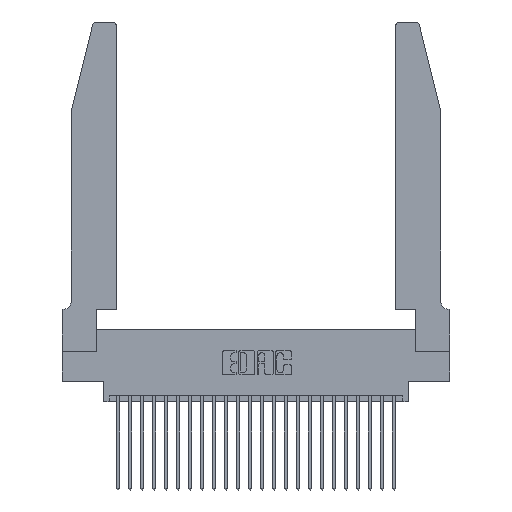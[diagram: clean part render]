
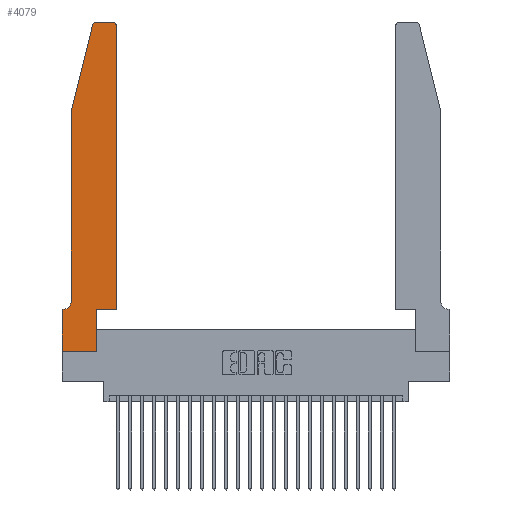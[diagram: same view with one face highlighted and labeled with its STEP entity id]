
A CAD part, top view. The second image highlights one B-rep face of the part: STEP entity #4079.
In plain terms, the highlighted planar face has unit normal (0, 0, 1).
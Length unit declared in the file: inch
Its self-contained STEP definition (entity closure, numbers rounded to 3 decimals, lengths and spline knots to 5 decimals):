
#277 = CIRCLE ( 'NONE', #853, 0.03 ) ;
#733 = CARTESIAN_POINT ( 'NONE',  ( 0.0755, 2., 0.37 ) ) ;
#740 = EDGE_CURVE ( 'NONE', #6446, #15986, #9805, .T. ) ;
#853 = AXIS2_PLACEMENT_3D ( 'NONE', #8101, #22144, #10156 ) ;
#1047 = LINE ( 'NONE', #12649, #11357 ) ;
#1340 = EDGE_CURVE ( 'NONE', #5785, #18816, #2372, .T. ) ;
#1494 = CARTESIAN_POINT ( 'NONE',  ( 0., 0., 0.37 ) ) ;
#1659 = LINE ( 'NONE', #18973, #11961 ) ;
#1955 = CARTESIAN_POINT ( 'NONE',  ( 0.4505, 2.72, 0.37 ) ) ;
#2372 = LINE ( 'NONE', #25134, #22603 ) ;
#2872 = CARTESIAN_POINT ( 'NONE',  ( 0.0755, 0.42, 0.37 ) ) ;
#3202 = CARTESIAN_POINT ( 'NONE',  ( 0., 0., 0.37 ) ) ;
#3206 = ORIENTED_EDGE ( 'NONE', *, *, #18783, .T. ) ;
#3615 = DIRECTION ( 'NONE',  ( 0., -1., 0. ) ) ;
#3975 = DIRECTION ( 'NONE',  ( 0., 0., -1. ) ) ;
#4079 = ADVANCED_FACE ( 'NONE', ( #21241 ), #5989, .T. ) ;
#4117 = EDGE_CURVE ( 'NONE', #4868, #4806, #277, .T. ) ;
#4322 = EDGE_CURVE ( 'NONE', #16030, #5785, #10305, .T. ) ;
#4368 = VECTOR ( 'NONE', #5799, 39.37008 ) ;
#4564 = CARTESIAN_POINT ( 'NONE',  ( 0.4205, 2.75, 0.37 ) ) ;
#4806 = VERTEX_POINT ( 'NONE', #12004 ) ;
#4868 = VERTEX_POINT ( 'NONE', #6229 ) ;
#5072 = AXIS2_PLACEMENT_3D ( 'NONE', #20044, #10072, #24035 ) ;
#5785 = VERTEX_POINT ( 'NONE', #21246 ) ;
#5799 = DIRECTION ( 'NONE',  ( 1., 0., 0. ) ) ;
#5846 = ORIENTED_EDGE ( 'NONE', *, *, #1340, .T. ) ;
#5989 = PLANE ( 'NONE',  #5072 ) ;
#6053 = CIRCLE ( 'NONE', #14151, 0.03 ) ;
#6054 = CARTESIAN_POINT ( 'NONE',  ( 0., 0.35, 0.37 ) ) ;
#6229 = CARTESIAN_POINT ( 'NONE',  ( 0.284, 2.75, 0.37 ) ) ;
#6446 = VERTEX_POINT ( 'NONE', #19137 ) ;
#6525 = DIRECTION ( 'NONE',  ( 1., 0., 0. ) ) ;
#6593 = EDGE_CURVE ( 'NONE', #18816, #8796, #6053, .T. ) ;
#7616 = VERTEX_POINT ( 'NONE', #2872 ) ;
#7746 = EDGE_CURVE ( 'NONE', #23694, #6446, #19477, .T. ) ;
#8046 = ORIENTED_EDGE ( 'NONE', *, *, #11347, .T. ) ;
#8101 = CARTESIAN_POINT ( 'NONE',  ( 0.284, 2.72, 0.37 ) ) ;
#8305 = LINE ( 'NONE', #14697, #18978 ) ;
#8796 = VERTEX_POINT ( 'NONE', #4564 ) ;
#8966 = CARTESIAN_POINT ( 'NONE',  ( 0.2865, 0., 0.37 ) ) ;
#9315 = ORIENTED_EDGE ( 'NONE', *, *, #7746, .T. ) ;
#9425 = VERTEX_POINT ( 'NONE', #733 ) ;
#9805 = LINE ( 'NONE', #3202, #4368 ) ;
#10072 = DIRECTION ( 'NONE',  ( 0., 0., 1. ) ) ;
#10156 = DIRECTION ( 'NONE',  ( 1., 0., 0. ) ) ;
#10305 = LINE ( 'NONE', #12724, #26183 ) ;
#11238 = ORIENTED_EDGE ( 'NONE', *, *, #6593, .T. ) ;
#11277 = CARTESIAN_POINT ( 'NONE',  ( 0.0755, 0.35, 0.37 ) ) ;
#11319 = CARTESIAN_POINT ( 'NONE',  ( 0.0055, 0.35, 0.37 ) ) ;
#11347 = EDGE_CURVE ( 'NONE', #4806, #9425, #8305, .T. ) ;
#11357 = VECTOR ( 'NONE', #24550, 39.37008 ) ;
#11543 = ORIENTED_EDGE ( 'NONE', *, *, #12066, .T. ) ;
#11635 = CARTESIAN_POINT ( 'NONE',  ( 0.4205, 2.72, 0.37 ) ) ;
#11961 = VECTOR ( 'NONE', #20966, 39.37008 ) ;
#12004 = CARTESIAN_POINT ( 'NONE',  ( 0.25487, 2.72718, 0.37 ) ) ;
#12066 = EDGE_CURVE ( 'NONE', #8796, #4868, #17994, .T. ) ;
#12649 = CARTESIAN_POINT ( 'NONE',  ( 0.2865, 0.35, 0.37 ) ) ;
#12724 = CARTESIAN_POINT ( 'NONE',  ( 0.4505, 0.35, 0.37 ) ) ;
#13315 = DIRECTION ( 'NONE',  ( -1., 0., 0. ) ) ;
#13664 = DIRECTION ( 'NONE',  ( 1., 0., 0. ) ) ;
#14151 = AXIS2_PLACEMENT_3D ( 'NONE', #11635, #25544, #13664 ) ;
#14176 = CIRCLE ( 'NONE', #18967, 0.07 ) ;
#14204 = VECTOR ( 'NONE', #3615, 39.37008 ) ;
#14697 = CARTESIAN_POINT ( 'NONE',  ( 0.0755, 2., 0.37 ) ) ;
#14754 = VECTOR ( 'NONE', #13315, 39.37008 ) ;
#15204 = CARTESIAN_POINT ( 'NONE',  ( 0.2865, 0.35, 0.37 ) ) ;
#15287 = ORIENTED_EDGE ( 'NONE', *, *, #4322, .T. ) ;
#15368 = LINE ( 'NONE', #11277, #14754 ) ;
#15986 = VERTEX_POINT ( 'NONE', #8966 ) ;
#16030 = VERTEX_POINT ( 'NONE', #15204 ) ;
#16101 = CARTESIAN_POINT ( 'NONE',  ( 0.0055, 0.42, 0.37 ) ) ;
#17360 = VECTOR ( 'NONE', #23202, 39.37008 ) ;
#17994 = LINE ( 'NONE', #21183, #17360 ) ;
#18010 = DIRECTION ( 'NONE',  ( 0., 1., 0. ) ) ;
#18109 = DIRECTION ( 'NONE',  ( -1., 0., 0. ) ) ;
#18726 = ORIENTED_EDGE ( 'NONE', *, *, #19118, .T. ) ;
#18783 = EDGE_CURVE ( 'NONE', #7616, #23015, #14176, .T. ) ;
#18791 = DIRECTION ( 'NONE',  ( -0.239, -0.971, 0. ) ) ;
#18816 = VERTEX_POINT ( 'NONE', #1955 ) ;
#18967 = AXIS2_PLACEMENT_3D ( 'NONE', #16101, #3975, #18109 ) ;
#18973 = CARTESIAN_POINT ( 'NONE',  ( 0.0755, 2., 0.37 ) ) ;
#18978 = VECTOR ( 'NONE', #18791, 39.37008 ) ;
#19118 = EDGE_CURVE ( 'NONE', #9425, #7616, #1659, .T. ) ;
#19137 = CARTESIAN_POINT ( 'NONE',  ( 0., 0., 0.37 ) ) ;
#19197 = EDGE_CURVE ( 'NONE', #23015, #23694, #15368, .T. ) ;
#19477 = LINE ( 'NONE', #1494, #14204 ) ;
#19989 = ORIENTED_EDGE ( 'NONE', *, *, #740, .T. ) ;
#20044 = CARTESIAN_POINT ( 'NONE',  ( 0., 0.35, 0.37 ) ) ;
#20966 = DIRECTION ( 'NONE',  ( 0., -1., 0. ) ) ;
#21183 = CARTESIAN_POINT ( 'NONE',  ( 0.2605, 2.75, 0.37 ) ) ;
#21241 = FACE_OUTER_BOUND ( 'NONE', #23861, .T. ) ;
#21246 = CARTESIAN_POINT ( 'NONE',  ( 0.4505, 0.35, 0.37 ) ) ;
#22144 = DIRECTION ( 'NONE',  ( 0., 0., 1. ) ) ;
#22171 = ORIENTED_EDGE ( 'NONE', *, *, #4117, .T. ) ;
#22603 = VECTOR ( 'NONE', #18010, 39.37008 ) ;
#23015 = VERTEX_POINT ( 'NONE', #11319 ) ;
#23202 = DIRECTION ( 'NONE',  ( -1., 0., 0. ) ) ;
#23694 = VERTEX_POINT ( 'NONE', #6054 ) ;
#23861 = EDGE_LOOP ( 'NONE', ( #11543, #22171, #8046, #18726, #3206, #24625, #9315, #19989, #25239, #15287, #5846, #11238 ) ) ;
#24035 = DIRECTION ( 'NONE',  ( 1., 0., 0. ) ) ;
#24550 = DIRECTION ( 'NONE',  ( 0., 1., 0. ) ) ;
#24625 = ORIENTED_EDGE ( 'NONE', *, *, #19197, .T. ) ;
#25067 = EDGE_CURVE ( 'NONE', #15986, #16030, #1047, .T. ) ;
#25134 = CARTESIAN_POINT ( 'NONE',  ( 0.4505, 0.35, 0.37 ) ) ;
#25239 = ORIENTED_EDGE ( 'NONE', *, *, #25067, .T. ) ;
#25544 = DIRECTION ( 'NONE',  ( 0., 0., 1. ) ) ;
#26183 = VECTOR ( 'NONE', #6525, 39.37008 ) ;
